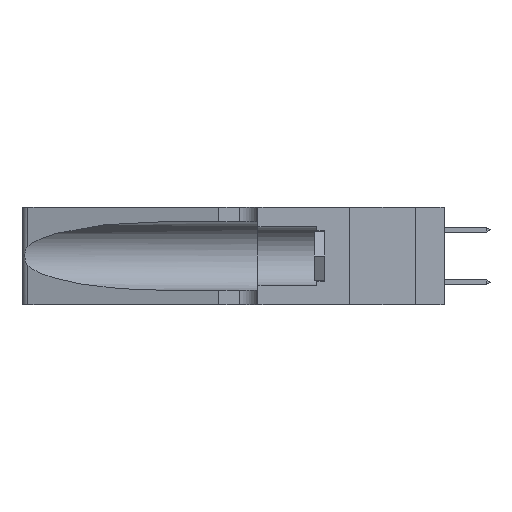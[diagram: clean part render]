
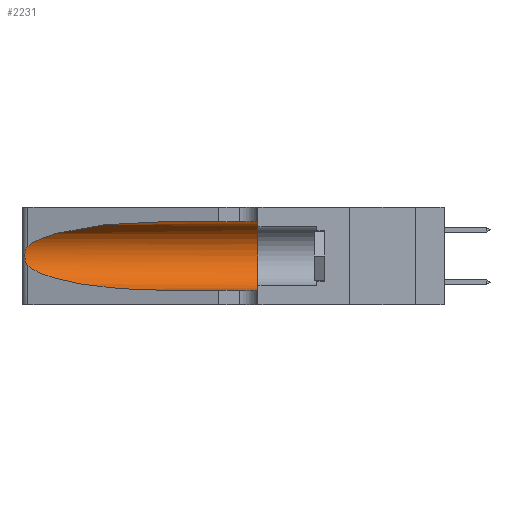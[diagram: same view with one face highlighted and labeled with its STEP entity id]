
A CAD part, left-side view. The second image highlights one B-rep face of the part: STEP entity #2231.
In plain terms, the highlighted cylindrical face has radius 3.308 mm (diameter 6.617 mm), a partial arc.
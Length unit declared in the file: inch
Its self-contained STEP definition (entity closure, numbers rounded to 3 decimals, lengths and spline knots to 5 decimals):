
#680 = EDGE_CURVE ( 'NONE', #16242, #14715, #13733, .T. ) ;
#794 = CARTESIAN_POINT ( 'NONE',  ( 0.1305, 0.35, 0.185 ) ) ;
#1581 = AXIS2_PLACEMENT_3D ( 'NONE', #794, #15059, #2865 ) ;
#2231 = ADVANCED_FACE ( 'NONE', ( #19735 ), #2859, .F. ) ;
#2600 = DIRECTION ( 'NONE',  ( 0., -1., 0. ) ) ;
#2859 = CYLINDRICAL_SURFACE ( 'NONE', #16353, 0.13025 ) ;
#2865 = DIRECTION ( 'NONE',  ( 0., 0., 1. ) ) ;
#3243 = CARTESIAN_POINT ( 'NONE',  ( 0.25787, 1.23484, 0.2124 ) ) ;
#3648 = ORIENTED_EDGE ( 'NONE', *, *, #680, .T. ) ;
#4158 = ORIENTED_EDGE ( 'NONE', *, *, #15559, .F. ) ;
#4477 = CARTESIAN_POINT ( 'NONE',  ( 0.25487, 1.22718, 0.22369 ) ) ;
#4605 = CARTESIAN_POINT ( 'NONE',  ( 0.25487, 1.22718, 0.14631 ) ) ;
#5323 = CARTESIAN_POINT ( 'NONE',  ( 0.26018, 1.23835, 0.19895 ) ) ;
#6414 = ORIENTED_EDGE ( 'NONE', *, *, #17065, .T. ) ;
#7399 = CARTESIAN_POINT ( 'NONE',  ( 0.26075, 1.23896, 0.178 ) ) ;
#7478 = VERTEX_POINT ( 'NONE', #4605 ) ;
#7747 = VECTOR ( 'NONE', #12105, 39.37008 ) ;
#8517 = ORIENTED_EDGE ( 'NONE', *, *, #24354, .F. ) ;
#9248 = CARTESIAN_POINT ( 'NONE',  ( 0.25487, 1.22718, 0.14631 ) ) ;
#9319 = CARTESIAN_POINT ( 'NONE',  ( 0.25487, 1.22718, 0.22369 ) ) ;
#9339 = CARTESIAN_POINT ( 'NONE',  ( 0.1305, 0.72297, 0.05475 ) ) ;
#9413 = CARTESIAN_POINT ( 'NONE',  ( 0.25856, 1.23593, 0.16098 ) ) ;
#9476 = EDGE_CURVE ( 'NONE', #7478, #16242, #11471, .T. ) ;
#9781 = CARTESIAN_POINT ( 'NONE',  ( 0.1305, 1.61858, 0.31525 ) ) ;
#10074 = CIRCLE ( 'NONE', #1581, 0.13025 ) ;
#10076 = CARTESIAN_POINT ( 'NONE',  ( 0.1305, 1.61858, 0.05475 ) ) ;
#10620 = VERTEX_POINT ( 'NONE', #23113 ) ;
#10922 = CARTESIAN_POINT ( 'NONE',  ( 0.1305, 0.72297, 0.05475 ) ) ;
#11420 = CARTESIAN_POINT ( 'NONE',  ( 0.25639, 1.23186, 0.15144 ) ) ;
#11471 =( BOUNDED_CURVE ( )  B_SPLINE_CURVE ( 3, ( #9248, #13304, #21499, #9339 ),
 .UNSPECIFIED., .F., .T. ) 
 B_SPLINE_CURVE_WITH_KNOTS ( ( 4, 4 ),
 ( 3.44316, 4.71239 ),
 .UNSPECIFIED. ) 
 CURVE ( )  GEOMETRIC_REPRESENTATION_ITEM ( )  RATIONAL_B_SPLINE_CURVE ( ( 1., 0.87, 0.87, 1. ) ) 
 REPRESENTATION_ITEM ( '' )  );
#11531 = CARTESIAN_POINT ( 'NONE',  ( 0.1305, 0.72297, 0.31525 ) ) ;
#11665 = ORIENTED_EDGE ( 'NONE', *, *, #25263, .T. ) ;
#12105 = DIRECTION ( 'NONE',  ( 0., -1., 0. ) ) ;
#12291 = LINE ( 'NONE', #9781, #23089 ) ;
#12294 =( BOUNDED_CURVE ( )  B_SPLINE_CURVE ( 3, ( #12561, #24682, #16652, #4477 ),
 .UNSPECIFIED., .F., .F. ) 
 B_SPLINE_CURVE_WITH_KNOTS ( ( 4, 4 ),
 ( 1.5708, 2.84003 ),
 .UNSPECIFIED. ) 
 CURVE ( )  GEOMETRIC_REPRESENTATION_ITEM ( )  RATIONAL_B_SPLINE_CURVE ( ( 1., 0.87, 0.87, 1. ) ) 
 REPRESENTATION_ITEM ( '' )  );
#12561 = CARTESIAN_POINT ( 'NONE',  ( 0.1305, 0.72297, 0.31525 ) ) ;
#12739 = CARTESIAN_POINT ( 'NONE',  ( 0.1305, 1.61858, 0.185 ) ) ;
#13304 = CARTESIAN_POINT ( 'NONE',  ( 0.2373, 1.15595, 0.08982 ) ) ;
#13467 = CARTESIAN_POINT ( 'NONE',  ( 0.25487, 1.22718, 0.14631 ) ) ;
#13733 = LINE ( 'NONE', #10076, #7747 ) ;
#14253 = B_SPLINE_CURVE_WITH_KNOTS ( 'NONE', 3,
 ( #9319, #21478, #15440, #3243, #17483, #5323, #19518, #7399, #21571, #9413, #23591, #11420, #25578, #13467 ),
 .UNSPECIFIED., .F., .F.,
 ( 4, 2, 2, 2, 2, 2, 4 ),
 ( 0., 0.00027, 0.00053, 0.00107, 0.0016, 0.00187, 0.00214 ),
 .UNSPECIFIED. ) ;
#14520 = CARTESIAN_POINT ( 'NONE',  ( 0.1305, 0.35, 0.05475 ) ) ;
#14715 = VERTEX_POINT ( 'NONE', #14520 ) ;
#14720 = DIRECTION ( 'NONE',  ( 0., 0., -1. ) ) ;
#15059 = DIRECTION ( 'NONE',  ( 0., 1., 0. ) ) ;
#15440 = CARTESIAN_POINT ( 'NONE',  ( 0.25639, 1.23184, 0.21858 ) ) ;
#15559 = EDGE_CURVE ( 'NONE', #10620, #14715, #10074, .T. ) ;
#15818 = EDGE_LOOP ( 'NONE', ( #11665, #6414, #22979, #3648, #4158, #8517 ) ) ;
#16242 = VERTEX_POINT ( 'NONE', #10922 ) ;
#16353 = AXIS2_PLACEMENT_3D ( 'NONE', #12739, #2600, #14720 ) ;
#16652 = CARTESIAN_POINT ( 'NONE',  ( 0.2373, 1.15595, 0.28018 ) ) ;
#17065 = EDGE_CURVE ( 'NONE', #23469, #7478, #14253, .T. ) ;
#17483 = CARTESIAN_POINT ( 'NONE',  ( 0.25854, 1.2359, 0.20912 ) ) ;
#19130 = CARTESIAN_POINT ( 'NONE',  ( 0.25487, 1.22718, 0.22369 ) ) ;
#19518 = CARTESIAN_POINT ( 'NONE',  ( 0.26075, 1.23896, 0.19203 ) ) ;
#19735 = FACE_OUTER_BOUND ( 'NONE', #15818, .T. ) ;
#21478 = CARTESIAN_POINT ( 'NONE',  ( 0.25555, 1.22994, 0.2215 ) ) ;
#21499 = CARTESIAN_POINT ( 'NONE',  ( 0.18966, 0.96281, 0.05475 ) ) ;
#21571 = CARTESIAN_POINT ( 'NONE',  ( 0.26017, 1.23833, 0.17102 ) ) ;
#22979 = ORIENTED_EDGE ( 'NONE', *, *, #9476, .T. ) ;
#23089 = VECTOR ( 'NONE', #23964, 39.37008 ) ;
#23113 = CARTESIAN_POINT ( 'NONE',  ( 0.1305, 0.35, 0.31525 ) ) ;
#23469 = VERTEX_POINT ( 'NONE', #19130 ) ;
#23591 = CARTESIAN_POINT ( 'NONE',  ( 0.25789, 1.23486, 0.15765 ) ) ;
#23964 = DIRECTION ( 'NONE',  ( 0., -1., 0. ) ) ;
#24298 = VERTEX_POINT ( 'NONE', #11531 ) ;
#24354 = EDGE_CURVE ( 'NONE', #24298, #10620, #12291, .T. ) ;
#24682 = CARTESIAN_POINT ( 'NONE',  ( 0.18966, 0.96281, 0.31525 ) ) ;
#25263 = EDGE_CURVE ( 'NONE', #24298, #23469, #12294, .T. ) ;
#25578 = CARTESIAN_POINT ( 'NONE',  ( 0.25555, 1.22993, 0.14849 ) ) ;
